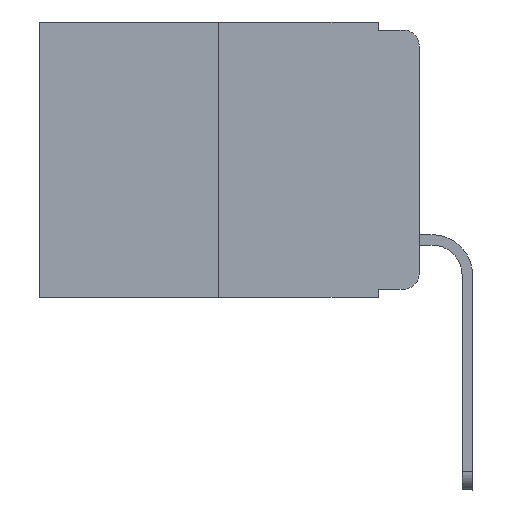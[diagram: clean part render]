
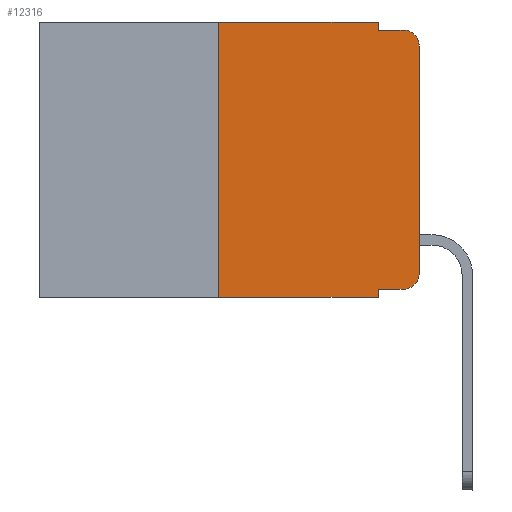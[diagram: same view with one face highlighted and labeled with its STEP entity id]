
A CAD part, left-side view. The second image highlights one B-rep face of the part: STEP entity #12316.
In plain terms, the highlighted planar face has unit normal (-1, 0, 0).
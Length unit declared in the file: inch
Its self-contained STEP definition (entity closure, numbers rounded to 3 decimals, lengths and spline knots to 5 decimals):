
#315 = LINE ( 'NONE', #8092, #3395 ) ;
#710 = CARTESIAN_POINT ( 'NONE',  ( 0., 0.02, -0.313 ) ) ;
#765 = AXIS2_PLACEMENT_3D ( 'NONE', #6551, #10019, #13831 ) ;
#877 = ORIENTED_EDGE ( 'NONE', *, *, #13229, .F. ) ;
#1092 = ORIENTED_EDGE ( 'NONE', *, *, #1956, .F. ) ;
#1225 = DIRECTION ( 'NONE',  ( 0., -1., 0. ) ) ;
#1426 = LINE ( 'NONE', #12429, #8185 ) ;
#1470 = CARTESIAN_POINT ( 'NONE',  ( 0., 0.473, 0. ) ) ;
#1956 = EDGE_CURVE ( 'NONE', #15808, #20432, #9879, .T. ) ;
#2218 = CIRCLE ( 'NONE', #14058, 0.02 ) ;
#2592 = DIRECTION ( 'NONE',  ( 0., 0., -1. ) ) ;
#2659 = VERTEX_POINT ( 'NONE', #16645 ) ;
#2739 = VECTOR ( 'NONE', #5058, 39.37008 ) ;
#3221 = DIRECTION ( 'NONE',  ( 0., 0., -1. ) ) ;
#3395 = VECTOR ( 'NONE', #22668, 39.37008 ) ;
#4529 = FACE_OUTER_BOUND ( 'NONE', #10640, .T. ) ;
#4644 = CARTESIAN_POINT ( 'NONE',  ( 0., 0.051, -0.01 ) ) ;
#4934 = LINE ( 'NONE', #19275, #6117 ) ;
#5014 = DIRECTION ( 'NONE',  ( -1., 0., 0. ) ) ;
#5058 = DIRECTION ( 'NONE',  ( 0., -1., 0. ) ) ;
#5193 = EDGE_CURVE ( 'NONE', #20432, #23122, #4934, .T. ) ;
#5362 = CARTESIAN_POINT ( 'NONE',  ( 0., 0.02, -0.03 ) ) ;
#5384 = CARTESIAN_POINT ( 'NONE',  ( 0., 0.051, -0.333 ) ) ;
#5418 = EDGE_CURVE ( 'NONE', #2659, #14196, #12806, .T. ) ;
#6117 = VECTOR ( 'NONE', #1225, 39.37008 ) ;
#6551 = CARTESIAN_POINT ( 'NONE',  ( 0., 0.473, 0. ) ) ;
#6606 = EDGE_CURVE ( 'NONE', #14983, #7253, #6841, .T. ) ;
#6608 = EDGE_CURVE ( 'NONE', #17397, #12360, #12348, .T. ) ;
#6620 = ORIENTED_EDGE ( 'NONE', *, *, #5193, .F. ) ;
#6841 = LINE ( 'NONE', #14129, #2739 ) ;
#7090 = ORIENTED_EDGE ( 'NONE', *, *, #8905, .T. ) ;
#7253 = VERTEX_POINT ( 'NONE', #9543 ) ;
#7654 = VECTOR ( 'NONE', #19622, 39.37008 ) ;
#7838 = CARTESIAN_POINT ( 'NONE',  ( 0., 0.051, -0.343 ) ) ;
#8092 = CARTESIAN_POINT ( 'NONE',  ( 0., 0.473, -0.343 ) ) ;
#8185 = VECTOR ( 'NONE', #3221, 39.37008 ) ;
#8437 = CARTESIAN_POINT ( 'NONE',  ( 0., 0.02, -0.01 ) ) ;
#8905 = EDGE_CURVE ( 'NONE', #2659, #18665, #315, .T. ) ;
#9026 = ORIENTED_EDGE ( 'NONE', *, *, #6608, .T. ) ;
#9271 = VECTOR ( 'NONE', #23345, 39.37008 ) ;
#9295 = ORIENTED_EDGE ( 'NONE', *, *, #10561, .T. ) ;
#9332 = CARTESIAN_POINT ( 'NONE',  ( 0., 0., 0. ) ) ;
#9543 = CARTESIAN_POINT ( 'NONE',  ( 0., 0.02, -0.333 ) ) ;
#9776 = PLANE ( 'NONE',  #765 ) ;
#9866 = AXIS2_PLACEMENT_3D ( 'NONE', #5362, #5014, #19468 ) ;
#9879 = LINE ( 'NONE', #19202, #23613 ) ;
#10019 = DIRECTION ( 'NONE',  ( 1., 0., 0. ) ) ;
#10525 = EDGE_CURVE ( 'NONE', #7253, #17397, #2218, .T. ) ;
#10561 = EDGE_CURVE ( 'NONE', #12360, #23122, #20170, .T. ) ;
#10640 = EDGE_LOOP ( 'NONE', ( #9026, #9295, #6620, #1092, #877, #12504, #7090, #20372, #18605, #11509 ) ) ;
#11509 = ORIENTED_EDGE ( 'NONE', *, *, #10525, .T. ) ;
#12316 = ADVANCED_FACE ( 'NONE', ( #4529 ), #9776, .F. ) ;
#12348 = LINE ( 'NONE', #9332, #22193 ) ;
#12360 = VERTEX_POINT ( 'NONE', #19930 ) ;
#12364 = CARTESIAN_POINT ( 'NONE',  ( 0., 0.051, 0. ) ) ;
#12429 = CARTESIAN_POINT ( 'NONE',  ( 0., 0.051, 0. ) ) ;
#12504 = ORIENTED_EDGE ( 'NONE', *, *, #5418, .F. ) ;
#12806 = LINE ( 'NONE', #21536, #7654 ) ;
#13208 = CARTESIAN_POINT ( 'NONE',  ( 0., 0., -0.313 ) ) ;
#13229 = EDGE_CURVE ( 'NONE', #14196, #15808, #19744, .T. ) ;
#13831 = DIRECTION ( 'NONE',  ( 0., 0., -1. ) ) ;
#14058 = AXIS2_PLACEMENT_3D ( 'NONE', #710, #20797, #18993 ) ;
#14129 = CARTESIAN_POINT ( 'NONE',  ( 0., 0.051, -0.333 ) ) ;
#14196 = VERTEX_POINT ( 'NONE', #20013 ) ;
#14983 = VERTEX_POINT ( 'NONE', #5384 ) ;
#15808 = VERTEX_POINT ( 'NONE', #12364 ) ;
#16645 = CARTESIAN_POINT ( 'NONE',  ( 0., 0.25, -0.343 ) ) ;
#17397 = VERTEX_POINT ( 'NONE', #13208 ) ;
#18081 = DIRECTION ( 'NONE',  ( 0., 0., 1. ) ) ;
#18605 = ORIENTED_EDGE ( 'NONE', *, *, #6606, .T. ) ;
#18665 = VERTEX_POINT ( 'NONE', #7838 ) ;
#18993 = DIRECTION ( 'NONE',  ( 0., 0., -1. ) ) ;
#19202 = CARTESIAN_POINT ( 'NONE',  ( 0., 0.051, 0. ) ) ;
#19275 = CARTESIAN_POINT ( 'NONE',  ( 0., 0.051, -0.01 ) ) ;
#19468 = DIRECTION ( 'NONE',  ( 0., 0., -1. ) ) ;
#19622 = DIRECTION ( 'NONE',  ( 0., 0., 1. ) ) ;
#19744 = LINE ( 'NONE', #1470, #9271 ) ;
#19930 = CARTESIAN_POINT ( 'NONE',  ( 0., 0., -0.03 ) ) ;
#20013 = CARTESIAN_POINT ( 'NONE',  ( 0., 0.25, 0. ) ) ;
#20077 = EDGE_CURVE ( 'NONE', #14983, #18665, #1426, .T. ) ;
#20170 = CIRCLE ( 'NONE', #9866, 0.02 ) ;
#20372 = ORIENTED_EDGE ( 'NONE', *, *, #20077, .F. ) ;
#20432 = VERTEX_POINT ( 'NONE', #4644 ) ;
#20797 = DIRECTION ( 'NONE',  ( -1., 0., 0. ) ) ;
#21536 = CARTESIAN_POINT ( 'NONE',  ( 0., 0.25, 0. ) ) ;
#22193 = VECTOR ( 'NONE', #18081, 39.37008 ) ;
#22668 = DIRECTION ( 'NONE',  ( 0., -1., 0. ) ) ;
#23122 = VERTEX_POINT ( 'NONE', #8437 ) ;
#23345 = DIRECTION ( 'NONE',  ( 0., -1., 0. ) ) ;
#23613 = VECTOR ( 'NONE', #2592, 39.37008 ) ;
